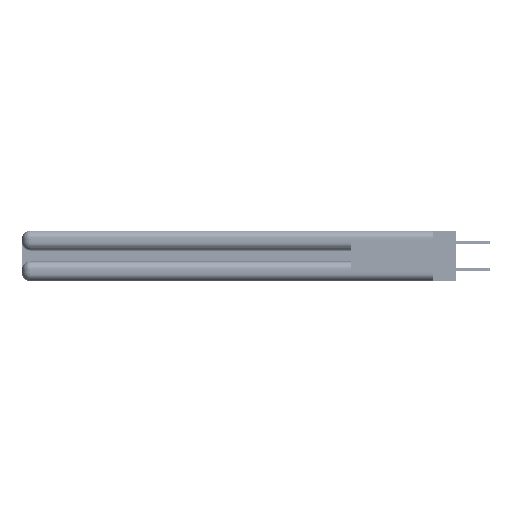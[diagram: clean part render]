
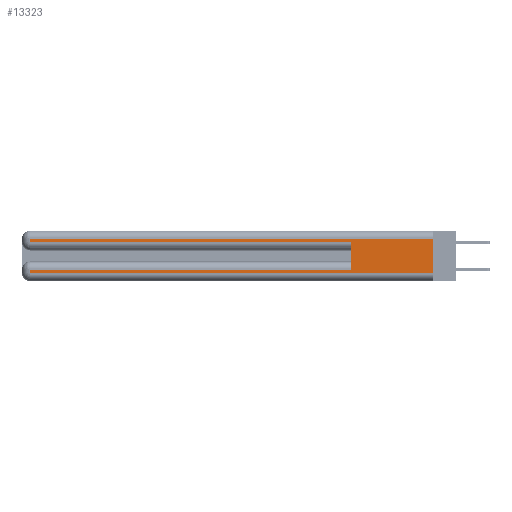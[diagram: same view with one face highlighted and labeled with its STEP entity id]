
A CAD part, left-side view. The second image highlights one B-rep face of the part: STEP entity #13323.
In plain terms, the highlighted planar face has unit normal (-1, 0, 0).
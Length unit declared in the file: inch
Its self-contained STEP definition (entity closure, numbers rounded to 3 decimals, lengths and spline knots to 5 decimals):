
#78 = VERTEX_POINT ( 'NONE', #24367 ) ;
#3701 = VERTEX_POINT ( 'NONE', #41836 ) ;
#3806 = FACE_OUTER_BOUND ( 'NONE', #13854, .T. ) ;
#4539 = LINE ( 'NONE', #28961, #33083 ) ;
#4911 = CARTESIAN_POINT ( 'NONE',  ( 0., 0., 0.085 ) ) ;
#5235 = CARTESIAN_POINT ( 'NONE',  ( 0., 0.6, 0.145 ) ) ;
#5269 = CARTESIAN_POINT ( 'NONE',  ( 0., 0., 0.37 ) ) ;
#5416 = PLANE ( 'NONE',  #22584 ) ;
#5721 = VECTOR ( 'NONE', #25452, 39.37008 ) ;
#6324 = DIRECTION ( 'NONE',  ( 0., 0., -1. ) ) ;
#6840 = LINE ( 'NONE', #43688, #39192 ) ;
#7719 = DIRECTION ( 'NONE',  ( 0., 1., 0. ) ) ;
#8274 = DIRECTION ( 'NONE',  ( 1., 0., 0. ) ) ;
#8463 = EDGE_CURVE ( 'NONE', #78, #22994, #24596, .T. ) ;
#10204 = EDGE_CURVE ( 'NONE', #3701, #11284, #6840, .T. ) ;
#11116 = VERTEX_POINT ( 'NONE', #36493 ) ;
#11206 = EDGE_CURVE ( 'NONE', #23001, #44314, #4539, .T. ) ;
#11284 = VERTEX_POINT ( 'NONE', #38602 ) ;
#11522 = VERTEX_POINT ( 'NONE', #23379 ) ;
#11859 = EDGE_CURVE ( 'NONE', #11116, #23001, #36888, .T. ) ;
#11910 = DIRECTION ( 'NONE',  ( 0., -1., 0. ) ) ;
#13323 = ADVANCED_FACE ( 'NONE', ( #3806 ), #5416, .F. ) ;
#13854 = EDGE_LOOP ( 'NONE', ( #16307, #20826, #41710, #14448, #17219, #14793, #14998, #26729 ) ) ;
#14106 = VECTOR ( 'NONE', #25628, 39.37008 ) ;
#14448 = ORIENTED_EDGE ( 'NONE', *, *, #20370, .T. ) ;
#14793 = ORIENTED_EDGE ( 'NONE', *, *, #44420, .T. ) ;
#14998 = ORIENTED_EDGE ( 'NONE', *, *, #11859, .T. ) ;
#15770 = VECTOR ( 'NONE', #34093, 39.37008 ) ;
#16305 = VECTOR ( 'NONE', #7719, 39.37008 ) ;
#16307 = ORIENTED_EDGE ( 'NONE', *, *, #25569, .F. ) ;
#17219 = ORIENTED_EDGE ( 'NONE', *, *, #8463, .F. ) ;
#17439 = LINE ( 'NONE', #32058, #14106 ) ;
#17919 = LINE ( 'NONE', #28770, #16305 ) ;
#20370 = EDGE_CURVE ( 'NONE', #11284, #22994, #17439, .T. ) ;
#20826 = ORIENTED_EDGE ( 'NONE', *, *, #38818, .T. ) ;
#22134 = DIRECTION ( 'NONE',  ( 0., 0., -1. ) ) ;
#22431 = VECTOR ( 'NONE', #26519, 39.37008 ) ;
#22584 = AXIS2_PLACEMENT_3D ( 'NONE', #5269, #8274, #29663 ) ;
#22994 = VERTEX_POINT ( 'NONE', #43795 ) ;
#23001 = VERTEX_POINT ( 'NONE', #24311 ) ;
#23379 = CARTESIAN_POINT ( 'NONE',  ( 0., 0., 0.31 ) ) ;
#24311 = CARTESIAN_POINT ( 'NONE',  ( 0., 2.94, 0.06 ) ) ;
#24367 = CARTESIAN_POINT ( 'NONE',  ( 0., 0.6, 0.085 ) ) ;
#24596 = LINE ( 'NONE', #5235, #15770 ) ;
#25452 = DIRECTION ( 'NONE',  ( 0., 1., 0. ) ) ;
#25569 = EDGE_CURVE ( 'NONE', #11522, #44314, #41185, .T. ) ;
#25628 = DIRECTION ( 'NONE',  ( 0., -1., 0. ) ) ;
#25912 = VECTOR ( 'NONE', #6324, 39.37008 ) ;
#26519 = DIRECTION ( 'NONE',  ( 0., 0., -1. ) ) ;
#26729 = ORIENTED_EDGE ( 'NONE', *, *, #11206, .T. ) ;
#28770 = CARTESIAN_POINT ( 'NONE',  ( 0., 0., 0.31 ) ) ;
#28961 = CARTESIAN_POINT ( 'NONE',  ( 0., 0., 0.06 ) ) ;
#29663 = DIRECTION ( 'NONE',  ( 0., 0., -1. ) ) ;
#29900 = LINE ( 'NONE', #4911, #5721 ) ;
#32058 = CARTESIAN_POINT ( 'NONE',  ( 0., 0., 0.285 ) ) ;
#32580 = CARTESIAN_POINT ( 'NONE',  ( 0., 0., 0.37 ) ) ;
#33083 = VECTOR ( 'NONE', #11910, 39.37008 ) ;
#33818 = CARTESIAN_POINT ( 'NONE',  ( 0., 2.94, 0.37 ) ) ;
#34093 = DIRECTION ( 'NONE',  ( 0., 0., 1. ) ) ;
#36493 = CARTESIAN_POINT ( 'NONE',  ( 0., 2.94, 0.085 ) ) ;
#36888 = LINE ( 'NONE', #33818, #25912 ) ;
#38602 = CARTESIAN_POINT ( 'NONE',  ( 0., 2.94, 0.285 ) ) ;
#38818 = EDGE_CURVE ( 'NONE', #11522, #3701, #17919, .T. ) ;
#39192 = VECTOR ( 'NONE', #22134, 39.37008 ) ;
#41185 = LINE ( 'NONE', #32580, #22431 ) ;
#41710 = ORIENTED_EDGE ( 'NONE', *, *, #10204, .T. ) ;
#41836 = CARTESIAN_POINT ( 'NONE',  ( 0., 2.94, 0.31 ) ) ;
#42362 = CARTESIAN_POINT ( 'NONE',  ( 0., 0., 0.06 ) ) ;
#43688 = CARTESIAN_POINT ( 'NONE',  ( 0., 2.94, 0.37 ) ) ;
#43795 = CARTESIAN_POINT ( 'NONE',  ( 0., 0.6, 0.285 ) ) ;
#44314 = VERTEX_POINT ( 'NONE', #42362 ) ;
#44420 = EDGE_CURVE ( 'NONE', #78, #11116, #29900, .T. ) ;
